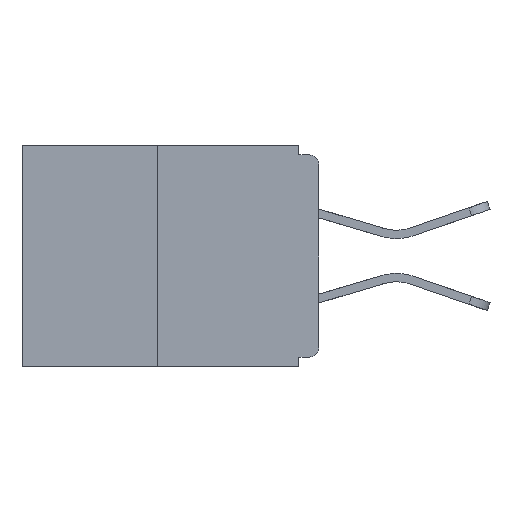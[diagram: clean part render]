
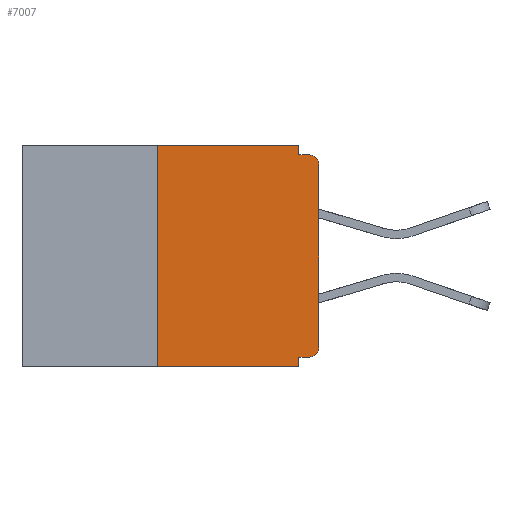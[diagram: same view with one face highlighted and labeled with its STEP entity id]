
A CAD part, left-side view. The second image highlights one B-rep face of the part: STEP entity #7007.
In plain terms, the highlighted planar face has unit normal (-1, 0, 0).
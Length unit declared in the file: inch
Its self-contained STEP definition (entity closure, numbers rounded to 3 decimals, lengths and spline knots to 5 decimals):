
#503 = CARTESIAN_POINT ( 'NONE',  ( 0., 0.031, -0.328 ) ) ;
#1363 = FACE_OUTER_BOUND ( 'NONE', #12198, .T. ) ;
#1452 = CARTESIAN_POINT ( 'NONE',  ( 0., 0.46, -0.343 ) ) ;
#1511 = ORIENTED_EDGE ( 'NONE', *, *, #15838, .F. ) ;
#1825 = VERTEX_POINT ( 'NONE', #8308 ) ;
#1882 = EDGE_CURVE ( 'NONE', #16589, #10068, #8667, .T. ) ;
#1905 = EDGE_CURVE ( 'NONE', #10018, #8526, #5442, .T. ) ;
#2031 = DIRECTION ( 'NONE',  ( 1., 0., 0. ) ) ;
#2052 = CARTESIAN_POINT ( 'NONE',  ( 0., 0.031, -0.343 ) ) ;
#2104 = ORIENTED_EDGE ( 'NONE', *, *, #9738, .T. ) ;
#2282 = CARTESIAN_POINT ( 'NONE',  ( 0., 0.25, 0. ) ) ;
#2322 = LINE ( 'NONE', #11943, #3579 ) ;
#2729 = VERTEX_POINT ( 'NONE', #503 ) ;
#2900 = DIRECTION ( 'NONE',  ( 0., -1., 0. ) ) ;
#3505 = PLANE ( 'NONE',  #16704 ) ;
#3568 = CARTESIAN_POINT ( 'NONE',  ( 0., 0.015, -0.313 ) ) ;
#3579 = VECTOR ( 'NONE', #10625, 39.37008 ) ;
#3666 = DIRECTION ( 'NONE',  ( 0., 0., -1. ) ) ;
#3680 = CIRCLE ( 'NONE', #14232, 0.015 ) ;
#4385 = CARTESIAN_POINT ( 'NONE',  ( 0., 0.031, -0.343 ) ) ;
#4442 = DIRECTION ( 'NONE',  ( 0., 0., -1. ) ) ;
#4556 = CARTESIAN_POINT ( 'NONE',  ( 0., 0.015, -0.015 ) ) ;
#4694 = ORIENTED_EDGE ( 'NONE', *, *, #6255, .F. ) ;
#4725 = DIRECTION ( 'NONE',  ( 0., 0., -1. ) ) ;
#4899 = DIRECTION ( 'NONE',  ( 0., 0., -1. ) ) ;
#5244 = LINE ( 'NONE', #4385, #15908 ) ;
#5442 = LINE ( 'NONE', #1452, #8035 ) ;
#5658 = LINE ( 'NONE', #13756, #6952 ) ;
#5748 = CARTESIAN_POINT ( 'NONE',  ( 0., 0.015, -0.328 ) ) ;
#6255 = EDGE_CURVE ( 'NONE', #2729, #8526, #5244, .T. ) ;
#6499 = EDGE_CURVE ( 'NONE', #10018, #16589, #5658, .T. ) ;
#6627 = EDGE_CURVE ( 'NONE', #6934, #1825, #16743, .T. ) ;
#6721 = VECTOR ( 'NONE', #2900, 39.37008 ) ;
#6934 = VERTEX_POINT ( 'NONE', #5748 ) ;
#6952 = VECTOR ( 'NONE', #7183, 39.37008 ) ;
#7007 = ADVANCED_FACE ( 'NONE', ( #1363 ), #3505, .F. ) ;
#7183 = DIRECTION ( 'NONE',  ( 0., 0., 1. ) ) ;
#7597 = VECTOR ( 'NONE', #17455, 39.37008 ) ;
#7722 = DIRECTION ( 'NONE',  ( -1., 0., 0. ) ) ;
#8035 = VECTOR ( 'NONE', #10840, 39.37008 ) ;
#8308 = CARTESIAN_POINT ( 'NONE',  ( 0., 0., -0.313 ) ) ;
#8526 = VERTEX_POINT ( 'NONE', #2052 ) ;
#8667 = LINE ( 'NONE', #11908, #6721 ) ;
#8846 = VERTEX_POINT ( 'NONE', #13920 ) ;
#9074 = AXIS2_PLACEMENT_3D ( 'NONE', #3568, #7722, #4899 ) ;
#9738 = EDGE_CURVE ( 'NONE', #8846, #11031, #3680, .T. ) ;
#9799 = LINE ( 'NONE', #10230, #10416 ) ;
#10018 = VERTEX_POINT ( 'NONE', #14142 ) ;
#10068 = VERTEX_POINT ( 'NONE', #10204 ) ;
#10152 = VERTEX_POINT ( 'NONE', #10375 ) ;
#10204 = CARTESIAN_POINT ( 'NONE',  ( 0., 0.031, 0. ) ) ;
#10230 = CARTESIAN_POINT ( 'NONE',  ( 0., 0.031, 0. ) ) ;
#10375 = CARTESIAN_POINT ( 'NONE',  ( 0., 0.031, -0.015 ) ) ;
#10377 = ORIENTED_EDGE ( 'NONE', *, *, #1882, .F. ) ;
#10416 = VECTOR ( 'NONE', #4725, 39.37008 ) ;
#10625 = DIRECTION ( 'NONE',  ( 0., -1., 0. ) ) ;
#10840 = DIRECTION ( 'NONE',  ( 0., -1., 0. ) ) ;
#11031 = VERTEX_POINT ( 'NONE', #4556 ) ;
#11191 = ORIENTED_EDGE ( 'NONE', *, *, #1905, .T. ) ;
#11438 = LINE ( 'NONE', #15998, #7597 ) ;
#11485 = LINE ( 'NONE', #12315, #16400 ) ;
#11908 = CARTESIAN_POINT ( 'NONE',  ( 0., 0.46, 0. ) ) ;
#11943 = CARTESIAN_POINT ( 'NONE',  ( 0., 0., -0.015 ) ) ;
#12198 = EDGE_LOOP ( 'NONE', ( #10377, #12642, #11191, #4694, #17330, #13801, #17076, #2104, #1511, #14807 ) ) ;
#12315 = CARTESIAN_POINT ( 'NONE',  ( 0., 0., 0. ) ) ;
#12642 = ORIENTED_EDGE ( 'NONE', *, *, #6499, .F. ) ;
#12754 = EDGE_CURVE ( 'NONE', #10068, #10152, #9799, .T. ) ;
#12828 = DIRECTION ( 'NONE',  ( 0., 0., -1. ) ) ;
#13061 = CARTESIAN_POINT ( 'NONE',  ( 0., 0.46, 0. ) ) ;
#13077 = EDGE_CURVE ( 'NONE', #1825, #8846, #11485, .T. ) ;
#13686 = DIRECTION ( 'NONE',  ( 0., 0., 1. ) ) ;
#13756 = CARTESIAN_POINT ( 'NONE',  ( 0., 0.25, 0. ) ) ;
#13801 = ORIENTED_EDGE ( 'NONE', *, *, #6627, .T. ) ;
#13920 = CARTESIAN_POINT ( 'NONE',  ( 0., 0., -0.03 ) ) ;
#14142 = CARTESIAN_POINT ( 'NONE',  ( 0., 0.25, -0.343 ) ) ;
#14232 = AXIS2_PLACEMENT_3D ( 'NONE', #16155, #14733, #3666 ) ;
#14733 = DIRECTION ( 'NONE',  ( -1., 0., 0. ) ) ;
#14807 = ORIENTED_EDGE ( 'NONE', *, *, #12754, .F. ) ;
#15442 = EDGE_CURVE ( 'NONE', #6934, #2729, #11438, .T. ) ;
#15838 = EDGE_CURVE ( 'NONE', #10152, #11031, #2322, .T. ) ;
#15908 = VECTOR ( 'NONE', #4442, 39.37008 ) ;
#15998 = CARTESIAN_POINT ( 'NONE',  ( 0., 0., -0.328 ) ) ;
#16155 = CARTESIAN_POINT ( 'NONE',  ( 0., 0.015, -0.03 ) ) ;
#16400 = VECTOR ( 'NONE', #13686, 39.37008 ) ;
#16589 = VERTEX_POINT ( 'NONE', #2282 ) ;
#16704 = AXIS2_PLACEMENT_3D ( 'NONE', #13061, #2031, #12828 ) ;
#16743 = CIRCLE ( 'NONE', #9074, 0.015 ) ;
#17076 = ORIENTED_EDGE ( 'NONE', *, *, #13077, .T. ) ;
#17330 = ORIENTED_EDGE ( 'NONE', *, *, #15442, .F. ) ;
#17455 = DIRECTION ( 'NONE',  ( 0., 1., 0. ) ) ;
